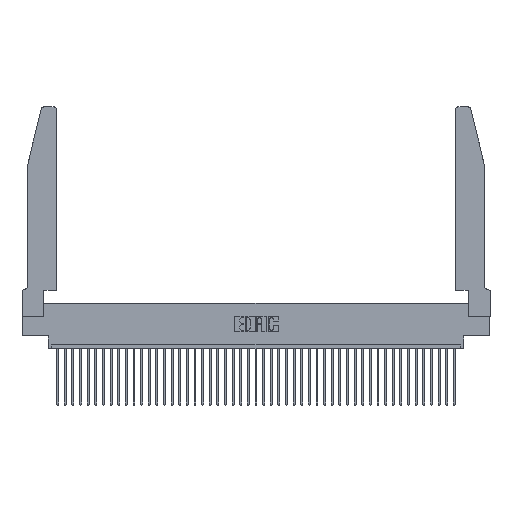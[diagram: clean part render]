
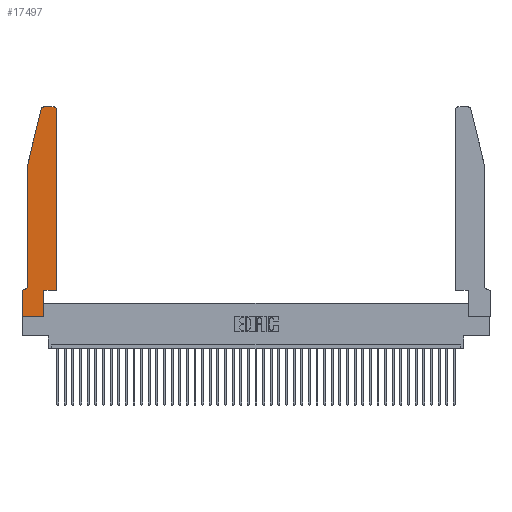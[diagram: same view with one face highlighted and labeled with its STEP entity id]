
A CAD part, top view. The second image highlights one B-rep face of the part: STEP entity #17497.
In plain terms, the highlighted planar face has unit normal (0, 0, 1).
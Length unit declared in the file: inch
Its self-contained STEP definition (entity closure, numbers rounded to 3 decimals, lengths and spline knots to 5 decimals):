
#1192 = EDGE_CURVE ( 'NONE', #26213, #36627, #37199, .T. ) ;
#2528 = AXIS2_PLACEMENT_3D ( 'NONE', #30163, #16960, #40421 ) ;
#2942 = CARTESIAN_POINT ( 'NONE',  ( 0.284, 2.72, 0.37 ) ) ;
#3245 = AXIS2_PLACEMENT_3D ( 'NONE', #20153, #36897, #30276 ) ;
#3627 = PLANE ( 'NONE',  #2528 ) ;
#3870 = CIRCLE ( 'NONE', #42449, 0.07 ) ;
#3919 = FACE_OUTER_BOUND ( 'NONE', #32311, .T. ) ;
#4192 = EDGE_CURVE ( 'NONE', #11709, #6168, #39875, .T. ) ;
#4507 = DIRECTION ( 'NONE',  ( 0., 1., 0. ) ) ;
#4925 = CARTESIAN_POINT ( 'NONE',  ( 0., 0., 0.37 ) ) ;
#5063 = ORIENTED_EDGE ( 'NONE', *, *, #22704, .T. ) ;
#5064 = CARTESIAN_POINT ( 'NONE',  ( 0.2865, 0.35, 0.37 ) ) ;
#5654 = VERTEX_POINT ( 'NONE', #23132 ) ;
#6040 = ORIENTED_EDGE ( 'NONE', *, *, #11219, .T. ) ;
#6168 = VERTEX_POINT ( 'NONE', #28787 ) ;
#7265 = DIRECTION ( 'NONE',  ( 1., 0., 0. ) ) ;
#7565 = CARTESIAN_POINT ( 'NONE',  ( 0.4505, 0.35, 0.37 ) ) ;
#7907 = CARTESIAN_POINT ( 'NONE',  ( 0.0055, 0.35, 0.37 ) ) ;
#8344 = ORIENTED_EDGE ( 'NONE', *, *, #32323, .T. ) ;
#8573 = EDGE_CURVE ( 'NONE', #12930, #35783, #40052, .T. ) ;
#11219 = EDGE_CURVE ( 'NONE', #36627, #14672, #27773, .T. ) ;
#11709 = VERTEX_POINT ( 'NONE', #4925 ) ;
#11833 = ORIENTED_EDGE ( 'NONE', *, *, #1192, .T. ) ;
#12132 = CARTESIAN_POINT ( 'NONE',  ( 0.4505, 2.72, 0.37 ) ) ;
#12157 = CARTESIAN_POINT ( 'NONE',  ( 0.0755, 2., 0.37 ) ) ;
#12439 = DIRECTION ( 'NONE',  ( 0., 0., -1. ) ) ;
#12930 = VERTEX_POINT ( 'NONE', #12132 ) ;
#13529 = CARTESIAN_POINT ( 'NONE',  ( 0., 0., 0.37 ) ) ;
#13656 = AXIS2_PLACEMENT_3D ( 'NONE', #2942, #26581, #40163 ) ;
#14672 = VERTEX_POINT ( 'NONE', #12157 ) ;
#14984 = ORIENTED_EDGE ( 'NONE', *, *, #22505, .T. ) ;
#15734 = CARTESIAN_POINT ( 'NONE',  ( 0.4205, 2.75, 0.37 ) ) ;
#16388 = CARTESIAN_POINT ( 'NONE',  ( 0.284, 2.75, 0.37 ) ) ;
#16765 = LINE ( 'NONE', #41050, #28683 ) ;
#16960 = DIRECTION ( 'NONE',  ( 0., 0., 1. ) ) ;
#17497 = ADVANCED_FACE ( 'NONE', ( #3919 ), #3627, .T. ) ;
#17534 = CARTESIAN_POINT ( 'NONE',  ( 0.25487, 2.72718, 0.37 ) ) ;
#17707 = VECTOR ( 'NONE', #4507, 39.37008 ) ;
#17845 = LINE ( 'NONE', #13529, #29294 ) ;
#18286 = LINE ( 'NONE', #32793, #20387 ) ;
#18384 = VECTOR ( 'NONE', #36324, 39.37008 ) ;
#20153 = CARTESIAN_POINT ( 'NONE',  ( 0.4205, 2.72, 0.37 ) ) ;
#20387 = VECTOR ( 'NONE', #7265, 39.37008 ) ;
#21224 = CARTESIAN_POINT ( 'NONE',  ( 0.4505, 0.35, 0.37 ) ) ;
#22167 = CARTESIAN_POINT ( 'NONE',  ( 0.0755, 0.42, 0.37 ) ) ;
#22505 = EDGE_CURVE ( 'NONE', #6168, #5654, #25082, .T. ) ;
#22704 = EDGE_CURVE ( 'NONE', #5654, #26591, #18286, .T. ) ;
#23132 = CARTESIAN_POINT ( 'NONE',  ( 0.2865, 0.35, 0.37 ) ) ;
#23147 = DIRECTION ( 'NONE',  ( 1., 0., 0. ) ) ;
#23348 = ORIENTED_EDGE ( 'NONE', *, *, #27722, .T. ) ;
#23779 = VECTOR ( 'NONE', #24477, 39.37008 ) ;
#23891 = ORIENTED_EDGE ( 'NONE', *, *, #38444, .T. ) ;
#24243 = VERTEX_POINT ( 'NONE', #34113 ) ;
#24477 = DIRECTION ( 'NONE',  ( -1., 0., 0. ) ) ;
#25082 = LINE ( 'NONE', #5064, #32851 ) ;
#25719 = ORIENTED_EDGE ( 'NONE', *, *, #4192, .T. ) ;
#25907 = EDGE_CURVE ( 'NONE', #32008, #30149, #3870, .T. ) ;
#26213 = VERTEX_POINT ( 'NONE', #16388 ) ;
#26401 = CARTESIAN_POINT ( 'NONE',  ( 0.0755, 2., 0.37 ) ) ;
#26581 = DIRECTION ( 'NONE',  ( 0., 0., 1. ) ) ;
#26591 = VERTEX_POINT ( 'NONE', #7565 ) ;
#26778 = VECTOR ( 'NONE', #32703, 39.37008 ) ;
#27722 = EDGE_CURVE ( 'NONE', #14672, #32008, #40807, .T. ) ;
#27773 = LINE ( 'NONE', #42287, #26778 ) ;
#28315 = ORIENTED_EDGE ( 'NONE', *, *, #25907, .T. ) ;
#28321 = VECTOR ( 'NONE', #23147, 39.37008 ) ;
#28683 = VECTOR ( 'NONE', #41482, 39.37008 ) ;
#28787 = CARTESIAN_POINT ( 'NONE',  ( 0.2865, 0., 0.37 ) ) ;
#29294 = VECTOR ( 'NONE', #36838, 39.37008 ) ;
#30070 = ORIENTED_EDGE ( 'NONE', *, *, #8573, .T. ) ;
#30149 = VERTEX_POINT ( 'NONE', #7907 ) ;
#30163 = CARTESIAN_POINT ( 'NONE',  ( 0., 0.35, 0.37 ) ) ;
#30276 = DIRECTION ( 'NONE',  ( 1., 0., 0. ) ) ;
#30968 = LINE ( 'NONE', #41415, #23779 ) ;
#32008 = VERTEX_POINT ( 'NONE', #22167 ) ;
#32311 = EDGE_LOOP ( 'NONE', ( #23891, #11833, #6040, #23348, #28315, #37215, #8344, #25719, #14984, #5063, #39048, #30070 ) ) ;
#32323 = EDGE_CURVE ( 'NONE', #24243, #11709, #17845, .T. ) ;
#32369 = CARTESIAN_POINT ( 'NONE',  ( 0.0055, 0.42, 0.37 ) ) ;
#32703 = DIRECTION ( 'NONE',  ( -0.239, -0.971, 0. ) ) ;
#32793 = CARTESIAN_POINT ( 'NONE',  ( 0.4505, 0.35, 0.37 ) ) ;
#32851 = VECTOR ( 'NONE', #39140, 39.37008 ) ;
#34113 = CARTESIAN_POINT ( 'NONE',  ( 0., 0.35, 0.37 ) ) ;
#35759 = DIRECTION ( 'NONE',  ( -1., 0., 0. ) ) ;
#35783 = VERTEX_POINT ( 'NONE', #15734 ) ;
#36324 = DIRECTION ( 'NONE',  ( 0., -1., 0. ) ) ;
#36627 = VERTEX_POINT ( 'NONE', #17534 ) ;
#36838 = DIRECTION ( 'NONE',  ( 0., -1., 0. ) ) ;
#36897 = DIRECTION ( 'NONE',  ( 0., 0., 1. ) ) ;
#37199 = CIRCLE ( 'NONE', #13656, 0.03 ) ;
#37215 = ORIENTED_EDGE ( 'NONE', *, *, #42316, .T. ) ;
#38444 = EDGE_CURVE ( 'NONE', #35783, #26213, #16765, .T. ) ;
#38585 = LINE ( 'NONE', #21224, #17707 ) ;
#39048 = ORIENTED_EDGE ( 'NONE', *, *, #40192, .T. ) ;
#39140 = DIRECTION ( 'NONE',  ( 0., 1., 0. ) ) ;
#39875 = LINE ( 'NONE', #40206, #28321 ) ;
#40052 = CIRCLE ( 'NONE', #3245, 0.03 ) ;
#40163 = DIRECTION ( 'NONE',  ( 1., 0., 0. ) ) ;
#40192 = EDGE_CURVE ( 'NONE', #26591, #12930, #38585, .T. ) ;
#40206 = CARTESIAN_POINT ( 'NONE',  ( 0., 0., 0.37 ) ) ;
#40421 = DIRECTION ( 'NONE',  ( 1., 0., 0. ) ) ;
#40807 = LINE ( 'NONE', #26401, #18384 ) ;
#41050 = CARTESIAN_POINT ( 'NONE',  ( 0.2605, 2.75, 0.37 ) ) ;
#41415 = CARTESIAN_POINT ( 'NONE',  ( 0.0755, 0.35, 0.37 ) ) ;
#41482 = DIRECTION ( 'NONE',  ( -1., 0., 0. ) ) ;
#42287 = CARTESIAN_POINT ( 'NONE',  ( 0.0755, 2., 0.37 ) ) ;
#42316 = EDGE_CURVE ( 'NONE', #30149, #24243, #30968, .T. ) ;
#42449 = AXIS2_PLACEMENT_3D ( 'NONE', #32369, #12439, #35759 ) ;
